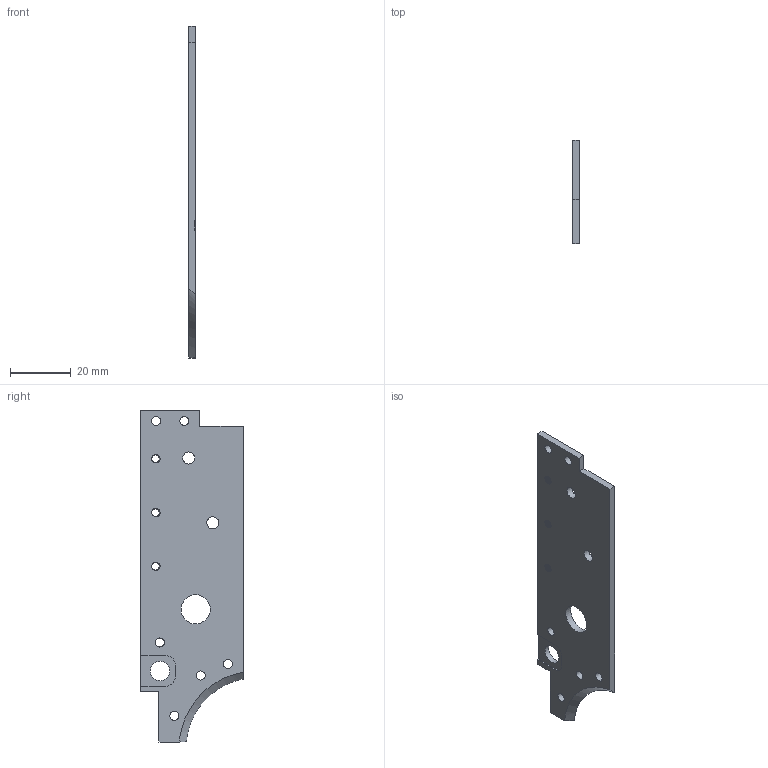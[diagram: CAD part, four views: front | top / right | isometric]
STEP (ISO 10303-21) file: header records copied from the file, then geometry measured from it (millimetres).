
FILE_DESCRIPTION(/* description */ (''),/* implementation_level */ '2;1');
FILE_NAME(/* name */ 'Rear SR Side Plate.step',/* time_stamp */ '2024-01-16T15:55:16-05:00',/* author */ (''),/* organization */ (''),/* preprocessor_version */ 'ST-DEVELOPER v20',/* originating_system */ 'Autodesk Translation Framework v12.14.0.127',/* authorisation */ '');
FILE_SCHEMA (('AUTOMOTIVE_DESIGN { 1 0 10303 214 3 1 1 }'));
Length unit declared in the file: inch
Products named in the file (1): Rear SR Side Plate
Bounding box: 2.29 x 33.91 x 109.73 mm (x, y, z)
Volume: 6886.6 mm3; surface area: 7126.3 mm2
Topology: 1 solids, 1 shells, 70 faces, 205 edges, 137 vertices
Faces by surface type: cylinder 46, plane 17, bspline 7
Full cylindrical faces by diameter (mm): 2.529 x3, 3 x6, 3.086 x3, 3.995 x2, 6.426 x1, 9.652 x1
Entity records: 4484 total; most frequent: CARTESIAN_POINT 2675, ORIENTED_EDGE 410, DIRECTION 288, EDGE_CURVE 205, VERTEX_POINT 137, AXIS2_PLACEMENT_3D 102, EDGE_LOOP 96, LINE 84
